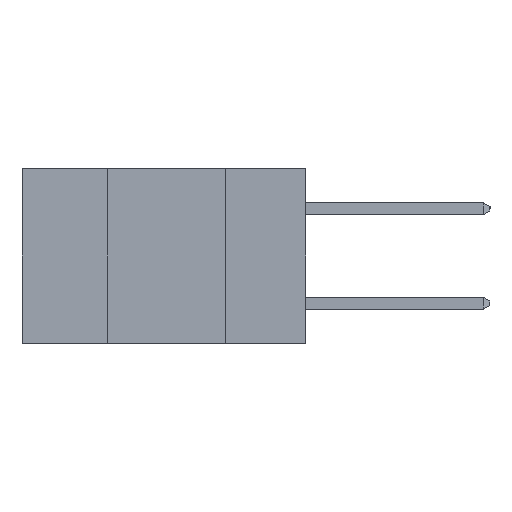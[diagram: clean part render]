
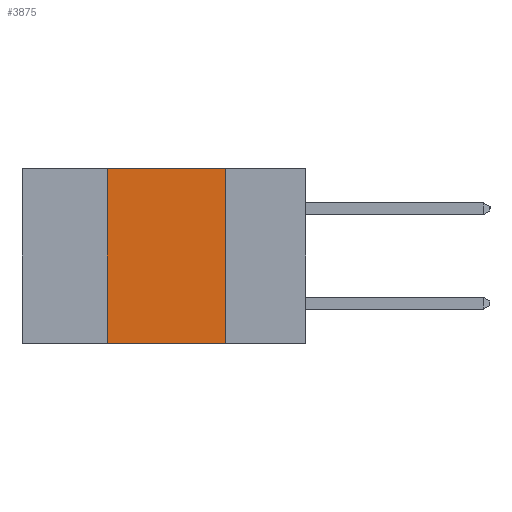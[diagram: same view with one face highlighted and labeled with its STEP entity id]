
A CAD part, left-side view. The second image highlights one B-rep face of the part: STEP entity #3875.
In plain terms, the highlighted planar face has unit normal (-1, 0, 0).
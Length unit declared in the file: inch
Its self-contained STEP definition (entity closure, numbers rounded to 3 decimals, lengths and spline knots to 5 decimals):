
#755 = AXIS2_PLACEMENT_3D ( 'NONE', #12595, #4577, #24816 ) ;
#1592 = EDGE_CURVE ( 'NONE', #14196, #3435, #21743, .T. ) ;
#1836 = ORIENTED_EDGE ( 'NONE', *, *, #22259, .T. ) ;
#3271 = VECTOR ( 'NONE', #19244, 39.37008 ) ;
#3435 = VERTEX_POINT ( 'NONE', #20346 ) ;
#3875 = ADVANCED_FACE ( 'NONE', ( #16895 ), #10523, .F. ) ;
#4037 = EDGE_CURVE ( 'NONE', #13542, #14196, #5336, .T. ) ;
#4531 = LINE ( 'NONE', #14769, #23961 ) ;
#4577 = DIRECTION ( 'NONE',  ( 1., 0., 0. ) ) ;
#5336 = LINE ( 'NONE', #11307, #3271 ) ;
#6611 = EDGE_CURVE ( 'NONE', #8129, #13542, #11957, .T. ) ;
#8129 = VERTEX_POINT ( 'NONE', #24421 ) ;
#10066 = CARTESIAN_POINT ( 'NONE',  ( 0., 0.17, -0.37 ) ) ;
#10233 = DIRECTION ( 'NONE',  ( 0., -1., 0. ) ) ;
#10356 = CARTESIAN_POINT ( 'NONE',  ( 0., 0.17, 0. ) ) ;
#10400 = VECTOR ( 'NONE', #20130, 39.37008 ) ;
#10523 = PLANE ( 'NONE',  #755 ) ;
#11307 = CARTESIAN_POINT ( 'NONE',  ( 0., 0.6, 0. ) ) ;
#11838 = EDGE_LOOP ( 'NONE', ( #12825, #16051, #23088, #1836 ) ) ;
#11957 = LINE ( 'NONE', #17956, #10400 ) ;
#12595 = CARTESIAN_POINT ( 'NONE',  ( 0., 0.6, 0. ) ) ;
#12825 = ORIENTED_EDGE ( 'NONE', *, *, #1592, .F. ) ;
#13542 = VERTEX_POINT ( 'NONE', #14462 ) ;
#14196 = VERTEX_POINT ( 'NONE', #10356 ) ;
#14462 = CARTESIAN_POINT ( 'NONE',  ( 0., 0.42, 0. ) ) ;
#14769 = CARTESIAN_POINT ( 'NONE',  ( 0., 0.6, -0.37 ) ) ;
#15684 = VECTOR ( 'NONE', #17993, 39.37008 ) ;
#16051 = ORIENTED_EDGE ( 'NONE', *, *, #4037, .F. ) ;
#16895 = FACE_OUTER_BOUND ( 'NONE', #11838, .T. ) ;
#17956 = CARTESIAN_POINT ( 'NONE',  ( 0., 0.42, -0.37 ) ) ;
#17993 = DIRECTION ( 'NONE',  ( 0., 0., -1. ) ) ;
#19244 = DIRECTION ( 'NONE',  ( 0., -1., 0. ) ) ;
#20130 = DIRECTION ( 'NONE',  ( 0., 0., 1. ) ) ;
#20346 = CARTESIAN_POINT ( 'NONE',  ( 0., 0.17, -0.37 ) ) ;
#21743 = LINE ( 'NONE', #10066, #15684 ) ;
#22259 = EDGE_CURVE ( 'NONE', #8129, #3435, #4531, .T. ) ;
#23088 = ORIENTED_EDGE ( 'NONE', *, *, #6611, .F. ) ;
#23961 = VECTOR ( 'NONE', #10233, 39.37008 ) ;
#24421 = CARTESIAN_POINT ( 'NONE',  ( 0., 0.42, -0.37 ) ) ;
#24816 = DIRECTION ( 'NONE',  ( 0., 0., -1. ) ) ;
